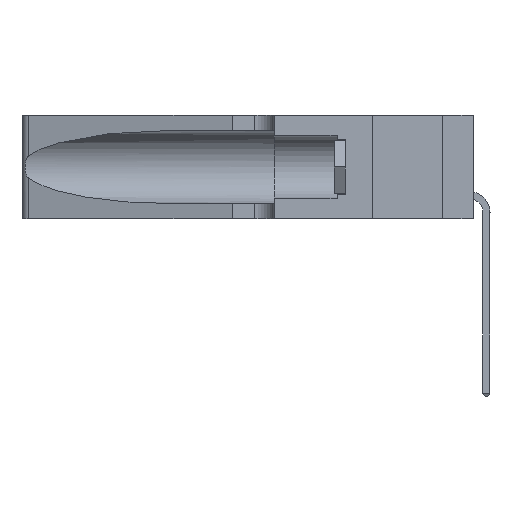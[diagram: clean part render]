
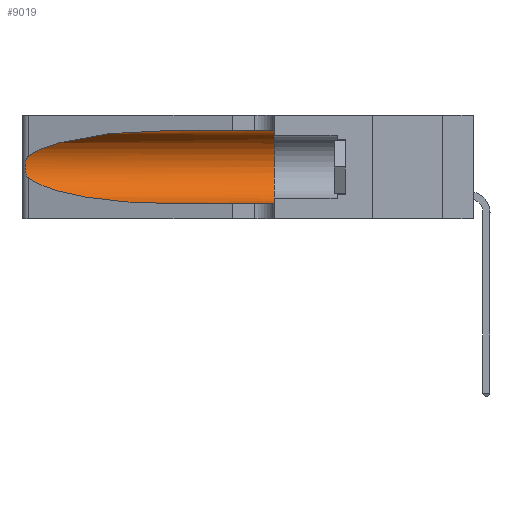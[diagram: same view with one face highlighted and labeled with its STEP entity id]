
A CAD part, left-side view. The second image highlights one B-rep face of the part: STEP entity #9019.
In plain terms, the highlighted cylindrical face has radius 3.308 mm (diameter 6.617 mm), a partial arc.
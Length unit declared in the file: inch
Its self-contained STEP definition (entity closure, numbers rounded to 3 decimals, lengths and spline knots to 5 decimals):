
#25 = CARTESIAN_POINT ( 'NONE',  ( 0.26075, 1.23896, 0.19203 ) ) ;
#825 = DIRECTION ( 'NONE',  ( 0., -1., 0. ) ) ;
#870 = CARTESIAN_POINT ( 'NONE',  ( 0.25787, 1.23484, 0.2124 ) ) ;
#1205 = EDGE_LOOP ( 'NONE', ( #21381, #16773, #10351, #17987, #15644, #13888 ) ) ;
#1448 = VECTOR ( 'NONE', #10295, 39.37008 ) ;
#1485 = EDGE_CURVE ( 'NONE', #14563, #15654, #9243, .T. ) ;
#1943 = CARTESIAN_POINT ( 'NONE',  ( 0.18966, 0.96281, 0.31525 ) ) ;
#2096 = CARTESIAN_POINT ( 'NONE',  ( 0.25487, 1.22718, 0.22369 ) ) ;
#2214 = LINE ( 'NONE', #3570, #1448 ) ;
#2523 = DIRECTION ( 'NONE',  ( 0., 0., -1. ) ) ;
#2917 = CIRCLE ( 'NONE', #19181, 0.13025 ) ;
#3570 = CARTESIAN_POINT ( 'NONE',  ( 0.1305, 1.61858, 0.05475 ) ) ;
#3728 = CARTESIAN_POINT ( 'NONE',  ( 0.1305, 0.35, 0.185 ) ) ;
#4030 = VERTEX_POINT ( 'NONE', #2096 ) ;
#4245 = EDGE_CURVE ( 'NONE', #4030, #21247, #17437, .T. ) ;
#4752 = CARTESIAN_POINT ( 'NONE',  ( 0.26017, 1.23833, 0.17102 ) ) ;
#4932 = EDGE_CURVE ( 'NONE', #15242, #19521, #2214, .T. ) ;
#4976 = CARTESIAN_POINT ( 'NONE',  ( 0.25854, 1.2359, 0.20912 ) ) ;
#5046 = CARTESIAN_POINT ( 'NONE',  ( 0.1305, 0.72297, 0.05475 ) ) ;
#5888 = CARTESIAN_POINT ( 'NONE',  ( 0.25639, 1.23186, 0.15144 ) ) ;
#6021 = EDGE_CURVE ( 'NONE', #14563, #4030, #7139, .T. ) ;
#7005 = CYLINDRICAL_SURFACE ( 'NONE', #16490, 0.13025 ) ;
#7061 = CARTESIAN_POINT ( 'NONE',  ( 0.25487, 1.22718, 0.14631 ) ) ;
#7139 =( BOUNDED_CURVE ( )  B_SPLINE_CURVE ( 3, ( #15174, #1943, #8618, #8456 ),
 .UNSPECIFIED., .F., .T. ) 
 B_SPLINE_CURVE_WITH_KNOTS ( ( 4, 4 ),
 ( 1.5708, 2.84003 ),
 .UNSPECIFIED. ) 
 CURVE ( )  GEOMETRIC_REPRESENTATION_ITEM ( )  RATIONAL_B_SPLINE_CURVE ( ( 1., 0.87, 0.87, 1. ) ) 
 REPRESENTATION_ITEM ( '' )  );
#8290 = CARTESIAN_POINT ( 'NONE',  ( 0.26018, 1.23835, 0.19895 ) ) ;
#8425 = CARTESIAN_POINT ( 'NONE',  ( 0.1305, 0.72297, 0.31525 ) ) ;
#8431 = VECTOR ( 'NONE', #825, 39.37008 ) ;
#8456 = CARTESIAN_POINT ( 'NONE',  ( 0.25487, 1.22718, 0.22369 ) ) ;
#8618 = CARTESIAN_POINT ( 'NONE',  ( 0.2373, 1.15595, 0.28018 ) ) ;
#8674 = CARTESIAN_POINT ( 'NONE',  ( 0.25856, 1.23593, 0.16098 ) ) ;
#9019 = ADVANCED_FACE ( 'NONE', ( #10915 ), #7005, .F. ) ;
#9223 = CARTESIAN_POINT ( 'NONE',  ( 0.25555, 1.22994, 0.2215 ) ) ;
#9243 = LINE ( 'NONE', #10986, #8431 ) ;
#9300 = CARTESIAN_POINT ( 'NONE',  ( 0.25487, 1.22718, 0.22369 ) ) ;
#10030 = CARTESIAN_POINT ( 'NONE',  ( 0.1305, 0.72297, 0.05475 ) ) ;
#10295 = DIRECTION ( 'NONE',  ( 0., -1., 0. ) ) ;
#10351 = ORIENTED_EDGE ( 'NONE', *, *, #15922, .T. ) ;
#10404 = DIRECTION ( 'NONE',  ( 0., 1., 0. ) ) ;
#10915 = FACE_OUTER_BOUND ( 'NONE', #1205, .T. ) ;
#10986 = CARTESIAN_POINT ( 'NONE',  ( 0.1305, 1.61858, 0.31525 ) ) ;
#12856 = EDGE_CURVE ( 'NONE', #15654, #19521, #2917, .T. ) ;
#13850 = DIRECTION ( 'NONE',  ( 0., 0., 1. ) ) ;
#13888 = ORIENTED_EDGE ( 'NONE', *, *, #1485, .F. ) ;
#14512 = DIRECTION ( 'NONE',  ( 0., -1., 0. ) ) ;
#14563 = VERTEX_POINT ( 'NONE', #8425 ) ;
#14781 = CARTESIAN_POINT ( 'NONE',  ( 0.2373, 1.15595, 0.08982 ) ) ;
#14863 = CARTESIAN_POINT ( 'NONE',  ( 0.26075, 1.23896, 0.178 ) ) ;
#15041 = CARTESIAN_POINT ( 'NONE',  ( 0.25789, 1.23486, 0.15765 ) ) ;
#15174 = CARTESIAN_POINT ( 'NONE',  ( 0.1305, 0.72297, 0.31525 ) ) ;
#15242 = VERTEX_POINT ( 'NONE', #10030 ) ;
#15530 = CARTESIAN_POINT ( 'NONE',  ( 0.1305, 0.35, 0.05475 ) ) ;
#15644 = ORIENTED_EDGE ( 'NONE', *, *, #12856, .F. ) ;
#15654 = VERTEX_POINT ( 'NONE', #16731 ) ;
#15853 = CARTESIAN_POINT ( 'NONE',  ( 0.25555, 1.22993, 0.14849 ) ) ;
#15922 = EDGE_CURVE ( 'NONE', #21247, #15242, #21013, .T. ) ;
#16490 = AXIS2_PLACEMENT_3D ( 'NONE', #21109, #14512, #2523 ) ;
#16731 = CARTESIAN_POINT ( 'NONE',  ( 0.1305, 0.35, 0.31525 ) ) ;
#16773 = ORIENTED_EDGE ( 'NONE', *, *, #4245, .T. ) ;
#17437 = B_SPLINE_CURVE_WITH_KNOTS ( 'NONE', 3,
 ( #9300, #9223, #20857, #870, #4976, #8290, #25, #14863, #4752, #8674, #15041, #5888, #15853, #19307 ),
 .UNSPECIFIED., .F., .F.,
 ( 4, 2, 2, 2, 2, 2, 4 ),
 ( 0., 0.00027, 0.00053, 0.00107, 0.0016, 0.00187, 0.00214 ),
 .UNSPECIFIED. ) ;
#17987 = ORIENTED_EDGE ( 'NONE', *, *, #4932, .T. ) ;
#18278 = CARTESIAN_POINT ( 'NONE',  ( 0.18966, 0.96281, 0.05475 ) ) ;
#19181 = AXIS2_PLACEMENT_3D ( 'NONE', #3728, #10404, #13850 ) ;
#19307 = CARTESIAN_POINT ( 'NONE',  ( 0.25487, 1.22718, 0.14631 ) ) ;
#19521 = VERTEX_POINT ( 'NONE', #15530 ) ;
#19803 = CARTESIAN_POINT ( 'NONE',  ( 0.25487, 1.22718, 0.14631 ) ) ;
#20857 = CARTESIAN_POINT ( 'NONE',  ( 0.25639, 1.23184, 0.21858 ) ) ;
#21013 =( BOUNDED_CURVE ( )  B_SPLINE_CURVE ( 3, ( #19803, #14781, #18278, #5046 ),
 .UNSPECIFIED., .F., .T. ) 
 B_SPLINE_CURVE_WITH_KNOTS ( ( 4, 4 ),
 ( 3.44316, 4.71239 ),
 .UNSPECIFIED. ) 
 CURVE ( )  GEOMETRIC_REPRESENTATION_ITEM ( )  RATIONAL_B_SPLINE_CURVE ( ( 1., 0.87, 0.87, 1. ) ) 
 REPRESENTATION_ITEM ( '' )  );
#21109 = CARTESIAN_POINT ( 'NONE',  ( 0.1305, 1.61858, 0.185 ) ) ;
#21247 = VERTEX_POINT ( 'NONE', #7061 ) ;
#21381 = ORIENTED_EDGE ( 'NONE', *, *, #6021, .T. ) ;
